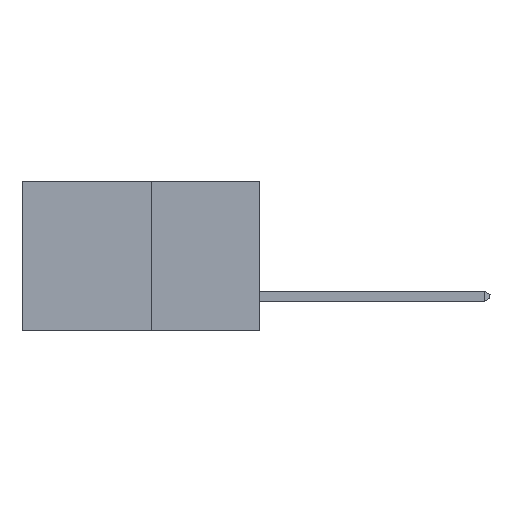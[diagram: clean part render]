
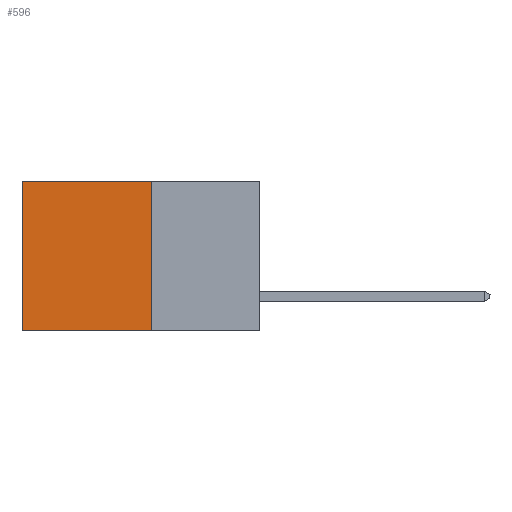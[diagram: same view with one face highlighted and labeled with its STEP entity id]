
A CAD part, left-side view. The second image highlights one B-rep face of the part: STEP entity #596.
In plain terms, the highlighted planar face has unit normal (-1, 0, 0).
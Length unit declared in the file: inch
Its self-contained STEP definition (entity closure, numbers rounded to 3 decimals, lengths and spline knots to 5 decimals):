
#596 = ADVANCED_FACE ( 'NONE', ( #4724 ), #2782, .F. ) ;
#1013 = LINE ( 'NONE', #5511, #4717 ) ;
#1385 = EDGE_CURVE ( 'NONE', #6821, #2475, #7886, .T. ) ;
#1705 = EDGE_LOOP ( 'NONE', ( #7203, #1955, #3885, #4117 ) ) ;
#1836 = VERTEX_POINT ( 'NONE', #5839 ) ;
#1955 = ORIENTED_EDGE ( 'NONE', *, *, #4209, .F. ) ;
#2013 = LINE ( 'NONE', #2101, #8574 ) ;
#2077 = DIRECTION ( 'NONE',  ( 0., 1., 0. ) ) ;
#2090 = LINE ( 'NONE', #2214, #3585 ) ;
#2101 = CARTESIAN_POINT ( 'NONE',  ( 0.277, 0.27, -0.37 ) ) ;
#2208 = DIRECTION ( 'NONE',  ( 0., 1., 0. ) ) ;
#2214 = CARTESIAN_POINT ( 'NONE',  ( 0.277, 0.27, 0. ) ) ;
#2475 = VERTEX_POINT ( 'NONE', #8616 ) ;
#2741 = VECTOR ( 'NONE', #4033, 39.37008 ) ;
#2782 = PLANE ( 'NONE',  #4348 ) ;
#2992 = VERTEX_POINT ( 'NONE', #6937 ) ;
#3585 = VECTOR ( 'NONE', #2208, 39.37008 ) ;
#3798 = CARTESIAN_POINT ( 'NONE',  ( 0.277, 0.27, -0.37 ) ) ;
#3885 = ORIENTED_EDGE ( 'NONE', *, *, #1385, .F. ) ;
#4015 = CARTESIAN_POINT ( 'NONE',  ( 0.277, 0.27, -0.37 ) ) ;
#4033 = DIRECTION ( 'NONE',  ( 0., 0., -1. ) ) ;
#4117 = ORIENTED_EDGE ( 'NONE', *, *, #6591, .T. ) ;
#4209 = EDGE_CURVE ( 'NONE', #2475, #1836, #2013, .T. ) ;
#4348 = AXIS2_PLACEMENT_3D ( 'NONE', #3798, #7191, #7202 ) ;
#4678 = EDGE_CURVE ( 'NONE', #2992, #1836, #1013, .T. ) ;
#4717 = VECTOR ( 'NONE', #5004, 39.37008 ) ;
#4724 = FACE_OUTER_BOUND ( 'NONE', #1705, .T. ) ;
#5004 = DIRECTION ( 'NONE',  ( 0., 0., -1. ) ) ;
#5511 = CARTESIAN_POINT ( 'NONE',  ( 0.277, 0.59, -0.37 ) ) ;
#5839 = CARTESIAN_POINT ( 'NONE',  ( 0.277, 0.59, -0.37 ) ) ;
#6591 = EDGE_CURVE ( 'NONE', #6821, #2992, #2090, .T. ) ;
#6821 = VERTEX_POINT ( 'NONE', #8472 ) ;
#6937 = CARTESIAN_POINT ( 'NONE',  ( 0.277, 0.59, 0. ) ) ;
#7191 = DIRECTION ( 'NONE',  ( 1., 0., 0. ) ) ;
#7202 = DIRECTION ( 'NONE',  ( 0., 0., -1. ) ) ;
#7203 = ORIENTED_EDGE ( 'NONE', *, *, #4678, .T. ) ;
#7886 = LINE ( 'NONE', #4015, #2741 ) ;
#8472 = CARTESIAN_POINT ( 'NONE',  ( 0.277, 0.27, 0. ) ) ;
#8574 = VECTOR ( 'NONE', #2077, 39.37008 ) ;
#8616 = CARTESIAN_POINT ( 'NONE',  ( 0.277, 0.27, -0.37 ) ) ;
